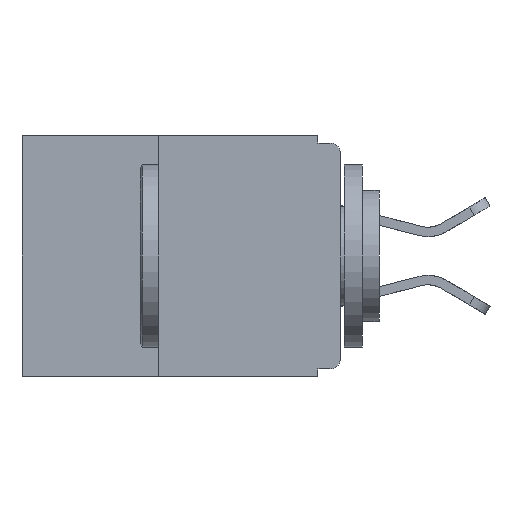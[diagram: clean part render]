
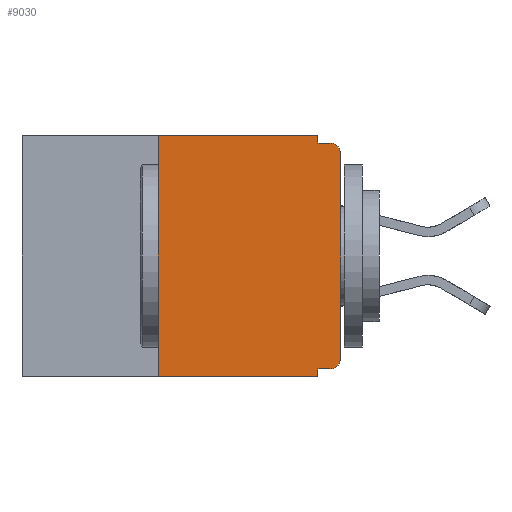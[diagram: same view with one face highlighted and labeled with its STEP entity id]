
A CAD part, left-side view. The second image highlights one B-rep face of the part: STEP entity #9030.
In plain terms, the highlighted planar face has unit normal (-1, 0, 0).
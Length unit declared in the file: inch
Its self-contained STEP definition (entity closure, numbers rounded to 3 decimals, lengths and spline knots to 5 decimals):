
#307 = ORIENTED_EDGE ( 'NONE', *, *, #10129, .T. ) ;
#332 = ORIENTED_EDGE ( 'NONE', *, *, #15750, .F. ) ;
#778 = EDGE_LOOP ( 'NONE', ( #14907, #307, #3394, #8420, #10526, #332, #5031, #13141, #7875, #3855 ) ) ;
#1002 = AXIS2_PLACEMENT_3D ( 'NONE', #4155, #4133, #4075 ) ;
#1105 = VERTEX_POINT ( 'NONE', #12441 ) ;
#1748 = VERTEX_POINT ( 'NONE', #3145 ) ;
#2245 = EDGE_CURVE ( 'NONE', #1105, #13390, #4287, .T. ) ;
#2590 = VERTEX_POINT ( 'NONE', #4713 ) ;
#3141 = EDGE_CURVE ( 'NONE', #9129, #18964, #8818, .T. ) ;
#3145 = CARTESIAN_POINT ( 'NONE',  ( 0., 0., -0.025 ) ) ;
#3181 = VECTOR ( 'NONE', #16229, 39.37008 ) ;
#3394 = ORIENTED_EDGE ( 'NONE', *, *, #11117, .F. ) ;
#3855 = ORIENTED_EDGE ( 'NONE', *, *, #13440, .T. ) ;
#3904 = CIRCLE ( 'NONE', #1002, 0.015 ) ;
#3945 = DIRECTION ( 'NONE',  ( 0., -1., 0. ) ) ;
#4075 = DIRECTION ( 'NONE',  ( 0., 0., -1. ) ) ;
#4133 = DIRECTION ( 'NONE',  ( -1., 0., 0. ) ) ;
#4155 = CARTESIAN_POINT ( 'NONE',  ( 0., 0.015, -0.025 ) ) ;
#4232 = CARTESIAN_POINT ( 'NONE',  ( 0., 0.031, -0.33 ) ) ;
#4287 = LINE ( 'NONE', #15432, #7325 ) ;
#4525 = CARTESIAN_POINT ( 'NONE',  ( 0., 0., -0.01 ) ) ;
#4713 = CARTESIAN_POINT ( 'NONE',  ( 0., 0.015, -0.32 ) ) ;
#4802 = VECTOR ( 'NONE', #3945, 39.37008 ) ;
#4900 = VECTOR ( 'NONE', #18892, 39.37008 ) ;
#5031 = ORIENTED_EDGE ( 'NONE', *, *, #3141, .T. ) ;
#5070 = CARTESIAN_POINT ( 'NONE',  ( 0., 0., -0.32 ) ) ;
#5318 = CARTESIAN_POINT ( 'NONE',  ( 0., 0.437, -0.33 ) ) ;
#5819 = LINE ( 'NONE', #8638, #16587 ) ;
#6033 = LINE ( 'NONE', #9619, #9535 ) ;
#6110 = CARTESIAN_POINT ( 'NONE',  ( 0., 0.015, -0.305 ) ) ;
#6557 = AXIS2_PLACEMENT_3D ( 'NONE', #16714, #16676, #16656 ) ;
#7316 = CARTESIAN_POINT ( 'NONE',  ( 0., 0.437, 0. ) ) ;
#7325 = VECTOR ( 'NONE', #10994, 39.37008 ) ;
#7443 = VERTEX_POINT ( 'NONE', #10021 ) ;
#7630 = DIRECTION ( 'NONE',  ( 0., 0., -1. ) ) ;
#7676 = LINE ( 'NONE', #10459, #3181 ) ;
#7875 = ORIENTED_EDGE ( 'NONE', *, *, #18784, .F. ) ;
#8143 = FACE_OUTER_BOUND ( 'NONE', #778, .T. ) ;
#8247 = VECTOR ( 'NONE', #16775, 39.37008 ) ;
#8420 = ORIENTED_EDGE ( 'NONE', *, *, #2245, .F. ) ;
#8629 = AXIS2_PLACEMENT_3D ( 'NONE', #6110, #16379, #7630 ) ;
#8638 = CARTESIAN_POINT ( 'NONE',  ( 0., 0., 0. ) ) ;
#8818 = LINE ( 'NONE', #5318, #13601 ) ;
#8890 = LINE ( 'NONE', #7316, #4900 ) ;
#9030 = ADVANCED_FACE ( 'NONE', ( #8143 ), #16892, .F. ) ;
#9129 = VERTEX_POINT ( 'NONE', #15562 ) ;
#9243 = VERTEX_POINT ( 'NONE', #14379 ) ;
#9535 = VECTOR ( 'NONE', #10030, 39.37008 ) ;
#9619 = CARTESIAN_POINT ( 'NONE',  ( 0., 0.031, -0.33 ) ) ;
#9698 = EDGE_CURVE ( 'NONE', #12048, #18964, #6033, .T. ) ;
#10021 = CARTESIAN_POINT ( 'NONE',  ( 0., 0.015, -0.01 ) ) ;
#10030 = DIRECTION ( 'NONE',  ( 0., 0., -1. ) ) ;
#10111 = DIRECTION ( 'NONE',  ( 0., 0., 1. ) ) ;
#10129 = EDGE_CURVE ( 'NONE', #1748, #7443, #3904, .T. ) ;
#10459 = CARTESIAN_POINT ( 'NONE',  ( 0., 0.25, -0.33 ) ) ;
#10526 = ORIENTED_EDGE ( 'NONE', *, *, #14515, .F. ) ;
#10994 = DIRECTION ( 'NONE',  ( 0., 0., -1. ) ) ;
#11117 = EDGE_CURVE ( 'NONE', #13390, #7443, #16512, .T. ) ;
#11663 = CIRCLE ( 'NONE', #8629, 0.015 ) ;
#11885 = CARTESIAN_POINT ( 'NONE',  ( 0., 0.031, -0.01 ) ) ;
#12048 = VERTEX_POINT ( 'NONE', #14074 ) ;
#12317 = DIRECTION ( 'NONE',  ( 0., -1., 0. ) ) ;
#12441 = CARTESIAN_POINT ( 'NONE',  ( 0., 0.031, 0. ) ) ;
#13141 = ORIENTED_EDGE ( 'NONE', *, *, #9698, .F. ) ;
#13218 = VERTEX_POINT ( 'NONE', #15271 ) ;
#13390 = VERTEX_POINT ( 'NONE', #11885 ) ;
#13440 = EDGE_CURVE ( 'NONE', #2590, #13218, #11663, .T. ) ;
#13601 = VECTOR ( 'NONE', #12317, 39.37008 ) ;
#14074 = CARTESIAN_POINT ( 'NONE',  ( 0., 0.031, -0.32 ) ) ;
#14379 = CARTESIAN_POINT ( 'NONE',  ( 0., 0.25, 0. ) ) ;
#14515 = EDGE_CURVE ( 'NONE', #9243, #1105, #8890, .T. ) ;
#14907 = ORIENTED_EDGE ( 'NONE', *, *, #14965, .T. ) ;
#14965 = EDGE_CURVE ( 'NONE', #13218, #1748, #5819, .T. ) ;
#15271 = CARTESIAN_POINT ( 'NONE',  ( 0., 0., -0.305 ) ) ;
#15432 = CARTESIAN_POINT ( 'NONE',  ( 0., 0.031, 0. ) ) ;
#15542 = LINE ( 'NONE', #5070, #8247 ) ;
#15562 = CARTESIAN_POINT ( 'NONE',  ( 0., 0.25, -0.33 ) ) ;
#15750 = EDGE_CURVE ( 'NONE', #9129, #9243, #7676, .T. ) ;
#16229 = DIRECTION ( 'NONE',  ( 0., 0., 1. ) ) ;
#16379 = DIRECTION ( 'NONE',  ( -1., 0., 0. ) ) ;
#16512 = LINE ( 'NONE', #4525, #4802 ) ;
#16587 = VECTOR ( 'NONE', #10111, 39.37008 ) ;
#16656 = DIRECTION ( 'NONE',  ( 0., 0., -1. ) ) ;
#16676 = DIRECTION ( 'NONE',  ( 1., 0., 0. ) ) ;
#16714 = CARTESIAN_POINT ( 'NONE',  ( 0., 0.437, 0. ) ) ;
#16775 = DIRECTION ( 'NONE',  ( 0., 1., 0. ) ) ;
#16892 = PLANE ( 'NONE',  #6557 ) ;
#18784 = EDGE_CURVE ( 'NONE', #2590, #12048, #15542, .T. ) ;
#18892 = DIRECTION ( 'NONE',  ( 0., -1., 0. ) ) ;
#18964 = VERTEX_POINT ( 'NONE', #4232 ) ;
